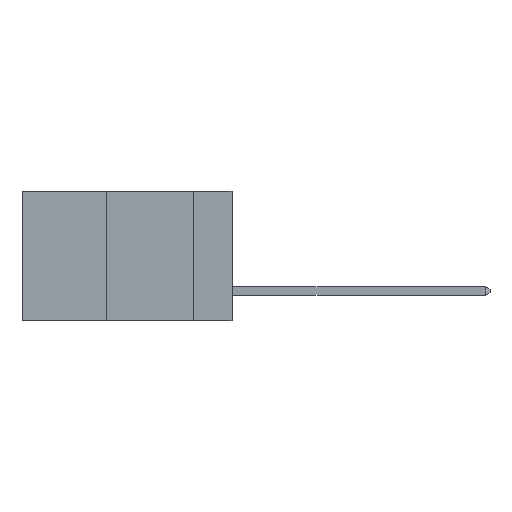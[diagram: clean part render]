
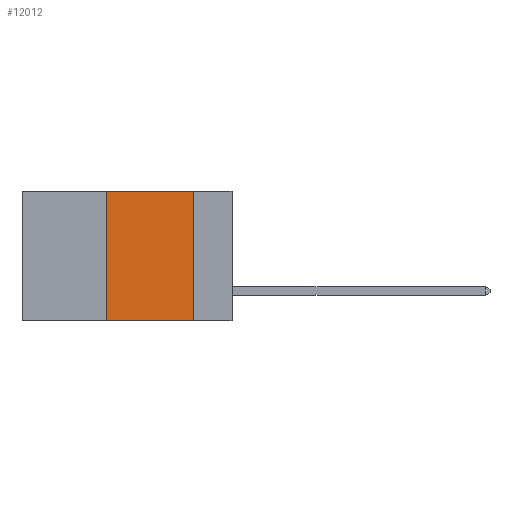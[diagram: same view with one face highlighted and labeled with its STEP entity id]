
A CAD part, left-side view. The second image highlights one B-rep face of the part: STEP entity #12012.
In plain terms, the highlighted planar face has unit normal (-1, 0, 0).
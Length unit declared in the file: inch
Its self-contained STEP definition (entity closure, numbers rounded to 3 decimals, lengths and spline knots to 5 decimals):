
#2088 = VERTEX_POINT ( 'NONE', #12259 ) ;
#2425 = CARTESIAN_POINT ( 'NONE',  ( 0., 0.6, -0.37 ) ) ;
#2990 = CARTESIAN_POINT ( 'NONE',  ( 0., 0.36, -0.37 ) ) ;
#3283 = LINE ( 'NONE', #28295, #26811 ) ;
#4613 = AXIS2_PLACEMENT_3D ( 'NONE', #26907, #29249, #15227 ) ;
#5775 = CARTESIAN_POINT ( 'NONE',  ( 0., 0.36, 0. ) ) ;
#6167 = VECTOR ( 'NONE', #19100, 39.37008 ) ;
#6359 = VERTEX_POINT ( 'NONE', #2990 ) ;
#6895 = EDGE_CURVE ( 'NONE', #6359, #18328, #14837, .T. ) ;
#7320 = DIRECTION ( 'NONE',  ( 0., -1., 0. ) ) ;
#8607 = VECTOR ( 'NONE', #7320, 39.37008 ) ;
#10111 = CARTESIAN_POINT ( 'NONE',  ( 0., 0.11, -0.37 ) ) ;
#12012 = ADVANCED_FACE ( 'NONE', ( #16091 ), #24564, .F. ) ;
#12251 = ORIENTED_EDGE ( 'NONE', *, *, #18854, .F. ) ;
#12259 = CARTESIAN_POINT ( 'NONE',  ( 0., 0.36, 0. ) ) ;
#12558 = ORIENTED_EDGE ( 'NONE', *, *, #19735, .F. ) ;
#12826 = LINE ( 'NONE', #5775, #25289 ) ;
#14837 = LINE ( 'NONE', #2425, #8607 ) ;
#15227 = DIRECTION ( 'NONE',  ( 0., 0., -1. ) ) ;
#16091 = FACE_OUTER_BOUND ( 'NONE', #27927, .T. ) ;
#18328 = VERTEX_POINT ( 'NONE', #10111 ) ;
#18633 = LINE ( 'NONE', #23729, #6167 ) ;
#18854 = EDGE_CURVE ( 'NONE', #24265, #18328, #3283, .T. ) ;
#19100 = DIRECTION ( 'NONE',  ( 0., -1., 0. ) ) ;
#19735 = EDGE_CURVE ( 'NONE', #6359, #2088, #12826, .T. ) ;
#19802 = DIRECTION ( 'NONE',  ( 0., 0., 1. ) ) ;
#22330 = EDGE_CURVE ( 'NONE', #2088, #24265, #18633, .T. ) ;
#23582 = DIRECTION ( 'NONE',  ( 0., 0., -1. ) ) ;
#23729 = CARTESIAN_POINT ( 'NONE',  ( 0., 0.6, 0. ) ) ;
#24265 = VERTEX_POINT ( 'NONE', #29522 ) ;
#24564 = PLANE ( 'NONE',  #4613 ) ;
#25289 = VECTOR ( 'NONE', #19802, 39.37008 ) ;
#26811 = VECTOR ( 'NONE', #23582, 39.37008 ) ;
#26907 = CARTESIAN_POINT ( 'NONE',  ( 0., 0.6, 0. ) ) ;
#27927 = EDGE_LOOP ( 'NONE', ( #12251, #30484, #12558, #28248 ) ) ;
#28248 = ORIENTED_EDGE ( 'NONE', *, *, #6895, .T. ) ;
#28295 = CARTESIAN_POINT ( 'NONE',  ( 0., 0.11, 0. ) ) ;
#29249 = DIRECTION ( 'NONE',  ( 1., 0., 0. ) ) ;
#29522 = CARTESIAN_POINT ( 'NONE',  ( 0., 0.11, 0. ) ) ;
#30484 = ORIENTED_EDGE ( 'NONE', *, *, #22330, .F. ) ;
